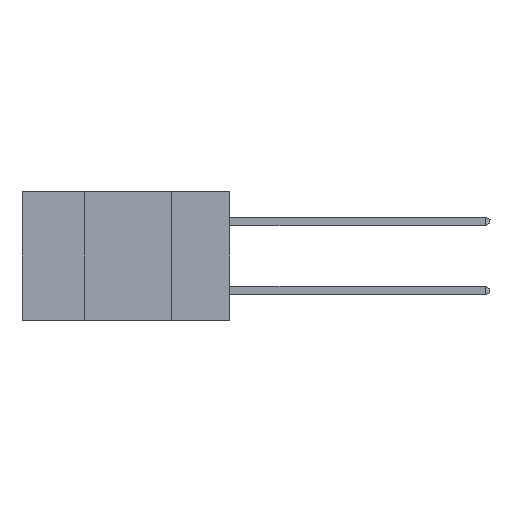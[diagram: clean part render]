
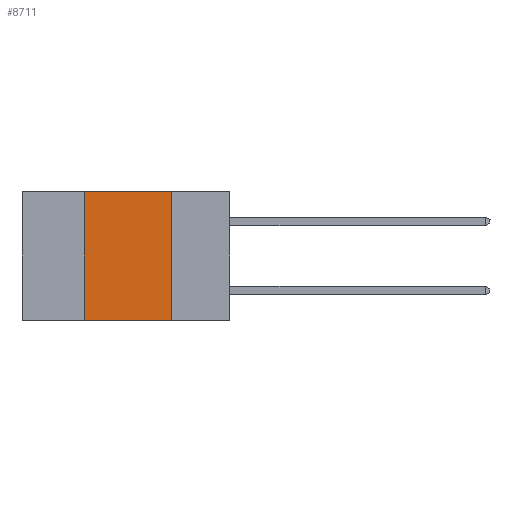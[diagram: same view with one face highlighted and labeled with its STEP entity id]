
A CAD part, left-side view. The second image highlights one B-rep face of the part: STEP entity #8711.
In plain terms, the highlighted planar face has unit normal (-1, 0, 0).
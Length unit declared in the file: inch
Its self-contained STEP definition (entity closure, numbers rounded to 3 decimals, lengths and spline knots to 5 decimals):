
#1331 = VECTOR ( 'NONE', #15276, 39.37008 ) ;
#1470 = EDGE_LOOP ( 'NONE', ( #7146, #5713, #18115, #3597 ) ) ;
#1970 = VECTOR ( 'NONE', #7516, 39.37008 ) ;
#2089 = EDGE_CURVE ( 'NONE', #18736, #4257, #18406, .T. ) ;
#2115 = DIRECTION ( 'NONE',  ( 1., 0., 0. ) ) ;
#2312 = CARTESIAN_POINT ( 'NONE',  ( 0., 0.6, -0.37 ) ) ;
#3597 = ORIENTED_EDGE ( 'NONE', *, *, #17263, .T. ) ;
#3740 = DIRECTION ( 'NONE',  ( 0., -1., 0. ) ) ;
#3981 = CARTESIAN_POINT ( 'NONE',  ( 0., 0.6, 0. ) ) ;
#4257 = VERTEX_POINT ( 'NONE', #7335 ) ;
#5571 = CARTESIAN_POINT ( 'NONE',  ( 0., 0.6, 0. ) ) ;
#5713 = ORIENTED_EDGE ( 'NONE', *, *, #16985, .F. ) ;
#7146 = ORIENTED_EDGE ( 'NONE', *, *, #12062, .F. ) ;
#7335 = CARTESIAN_POINT ( 'NONE',  ( 0., 0.42, 0. ) ) ;
#7516 = DIRECTION ( 'NONE',  ( 0., 0., 1. ) ) ;
#7613 = LINE ( 'NONE', #14916, #1331 ) ;
#8711 = ADVANCED_FACE ( 'NONE', ( #21686 ), #10817, .F. ) ;
#9572 = DIRECTION ( 'NONE',  ( 0., -1., 0. ) ) ;
#10258 = CARTESIAN_POINT ( 'NONE',  ( 0., 0.17, -0.37 ) ) ;
#10817 = PLANE ( 'NONE',  #13877 ) ;
#11722 = VERTEX_POINT ( 'NONE', #10258 ) ;
#12062 = EDGE_CURVE ( 'NONE', #22846, #11722, #7613, .T. ) ;
#13877 = AXIS2_PLACEMENT_3D ( 'NONE', #5571, #2115, #18252 ) ;
#13919 = VECTOR ( 'NONE', #9572, 39.37008 ) ;
#14916 = CARTESIAN_POINT ( 'NONE',  ( 0., 0.17, -0.37 ) ) ;
#15235 = CARTESIAN_POINT ( 'NONE',  ( 0., 0.17, 0. ) ) ;
#15276 = DIRECTION ( 'NONE',  ( 0., 0., -1. ) ) ;
#16985 = EDGE_CURVE ( 'NONE', #4257, #22846, #18569, .T. ) ;
#17263 = EDGE_CURVE ( 'NONE', #18736, #11722, #17355, .T. ) ;
#17355 = LINE ( 'NONE', #2312, #13919 ) ;
#17436 = CARTESIAN_POINT ( 'NONE',  ( 0., 0.42, -0.37 ) ) ;
#18115 = ORIENTED_EDGE ( 'NONE', *, *, #2089, .F. ) ;
#18252 = DIRECTION ( 'NONE',  ( 0., 0., -1. ) ) ;
#18406 = LINE ( 'NONE', #20190, #1970 ) ;
#18569 = LINE ( 'NONE', #3981, #21515 ) ;
#18736 = VERTEX_POINT ( 'NONE', #17436 ) ;
#20190 = CARTESIAN_POINT ( 'NONE',  ( 0., 0.42, -0.37 ) ) ;
#21515 = VECTOR ( 'NONE', #3740, 39.37008 ) ;
#21686 = FACE_OUTER_BOUND ( 'NONE', #1470, .T. ) ;
#22846 = VERTEX_POINT ( 'NONE', #15235 ) ;
